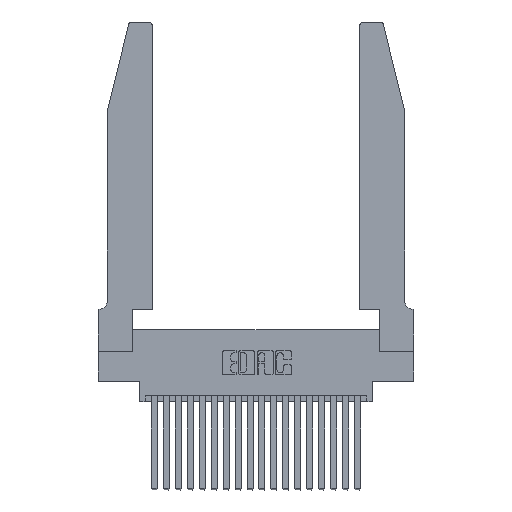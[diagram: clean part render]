
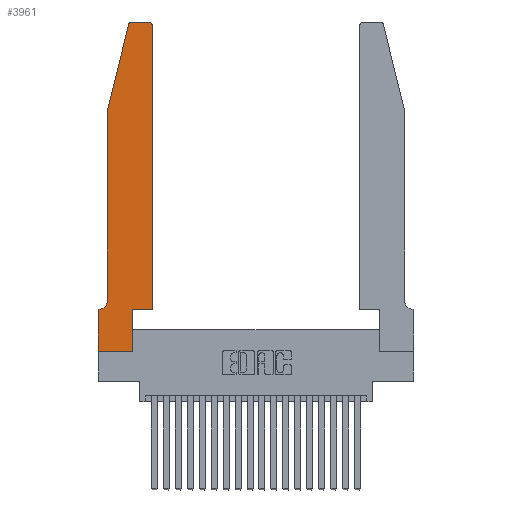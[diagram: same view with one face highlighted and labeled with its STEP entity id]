
A CAD part, top view. The second image highlights one B-rep face of the part: STEP entity #3961.
In plain terms, the highlighted planar face has unit normal (0, 0, 1).
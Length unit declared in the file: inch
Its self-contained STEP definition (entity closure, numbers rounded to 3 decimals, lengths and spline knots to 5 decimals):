
#35 = EDGE_CURVE ( 'NONE', #13079, #6529, #223, .T. ) ;
#199 = DIRECTION ( 'NONE',  ( -0.239, -0.971, 0. ) ) ;
#223 = LINE ( 'NONE', #14886, #17971 ) ;
#735 = CIRCLE ( 'NONE', #3611, 0.07 ) ;
#894 = ORIENTED_EDGE ( 'NONE', *, *, #7632, .T. ) ;
#1057 = VERTEX_POINT ( 'NONE', #8430 ) ;
#1922 = DIRECTION ( 'NONE',  ( -1., 0., 0. ) ) ;
#2214 = LINE ( 'NONE', #8737, #18804 ) ;
#2831 = CARTESIAN_POINT ( 'NONE',  ( 0.2865, 0.35, 0.37 ) ) ;
#2945 = CARTESIAN_POINT ( 'NONE',  ( 0.0755, 2., 0.37 ) ) ;
#3165 = DIRECTION ( 'NONE',  ( 0., 0., 1. ) ) ;
#3611 = AXIS2_PLACEMENT_3D ( 'NONE', #7350, #19250, #9054 ) ;
#3693 = CIRCLE ( 'NONE', #13546, 0.03 ) ;
#3961 = ADVANCED_FACE ( 'NONE', ( #19133 ), #3988, .T. ) ;
#3988 = PLANE ( 'NONE',  #6162 ) ;
#4061 = LINE ( 'NONE', #18383, #12732 ) ;
#4162 = CARTESIAN_POINT ( 'NONE',  ( 0.0055, 0.35, 0.37 ) ) ;
#4624 = CARTESIAN_POINT ( 'NONE',  ( 0., 0., 0.37 ) ) ;
#5386 = CARTESIAN_POINT ( 'NONE',  ( 0.4205, 2.72, 0.37 ) ) ;
#5396 = ORIENTED_EDGE ( 'NONE', *, *, #18853, .T. ) ;
#5871 = CARTESIAN_POINT ( 'NONE',  ( 0.0755, 0.42, 0.37 ) ) ;
#5880 = LINE ( 'NONE', #20763, #18961 ) ;
#6095 = ORIENTED_EDGE ( 'NONE', *, *, #13916, .T. ) ;
#6162 = AXIS2_PLACEMENT_3D ( 'NONE', #16023, #17713, #7493 ) ;
#6344 = EDGE_CURVE ( 'NONE', #21919, #13079, #7239, .T. ) ;
#6529 = VERTEX_POINT ( 'NONE', #12059 ) ;
#6833 = ORIENTED_EDGE ( 'NONE', *, *, #9763, .T. ) ;
#7139 = DIRECTION ( 'NONE',  ( 1., 0., 0. ) ) ;
#7226 = VERTEX_POINT ( 'NONE', #10569 ) ;
#7239 = LINE ( 'NONE', #4624, #15816 ) ;
#7350 = CARTESIAN_POINT ( 'NONE',  ( 0.0055, 0.42, 0.37 ) ) ;
#7493 = DIRECTION ( 'NONE',  ( 1., 0., 0. ) ) ;
#7632 = EDGE_CURVE ( 'NONE', #1057, #8262, #18911, .T. ) ;
#7889 = VERTEX_POINT ( 'NONE', #17749 ) ;
#8262 = VERTEX_POINT ( 'NONE', #20699 ) ;
#8427 = VECTOR ( 'NONE', #17951, 39.37008 ) ;
#8430 = CARTESIAN_POINT ( 'NONE',  ( 0.284, 2.75, 0.37 ) ) ;
#8674 = ORIENTED_EDGE ( 'NONE', *, *, #17031, .T. ) ;
#8737 = CARTESIAN_POINT ( 'NONE',  ( 0.0755, 2., 0.37 ) ) ;
#8948 = CARTESIAN_POINT ( 'NONE',  ( 0.4205, 2.75, 0.37 ) ) ;
#8961 = VERTEX_POINT ( 'NONE', #5871 ) ;
#9054 = DIRECTION ( 'NONE',  ( -1., 0., 0. ) ) ;
#9763 = EDGE_CURVE ( 'NONE', #18347, #1057, #19605, .T. ) ;
#10079 = DIRECTION ( 'NONE',  ( -1., 0., 0. ) ) ;
#10315 = VERTEX_POINT ( 'NONE', #4162 ) ;
#10489 = DIRECTION ( 'NONE',  ( 0., -1., 0. ) ) ;
#10569 = CARTESIAN_POINT ( 'NONE',  ( 0.4505, 0.35, 0.37 ) ) ;
#10728 = LINE ( 'NONE', #18016, #19208 ) ;
#10960 = ORIENTED_EDGE ( 'NONE', *, *, #14172, .T. ) ;
#11254 = EDGE_CURVE ( 'NONE', #21635, #8961, #2214, .T. ) ;
#12022 = ORIENTED_EDGE ( 'NONE', *, *, #6344, .T. ) ;
#12059 = CARTESIAN_POINT ( 'NONE',  ( 0.2865, 0., 0.37 ) ) ;
#12732 = VECTOR ( 'NONE', #21693, 39.37008 ) ;
#13079 = VERTEX_POINT ( 'NONE', #15559 ) ;
#13095 = ORIENTED_EDGE ( 'NONE', *, *, #35, .T. ) ;
#13500 = CARTESIAN_POINT ( 'NONE',  ( 0.284, 2.72, 0.37 ) ) ;
#13546 = AXIS2_PLACEMENT_3D ( 'NONE', #5386, #17365, #7139 ) ;
#13916 = EDGE_CURVE ( 'NONE', #20949, #7226, #21890, .T. ) ;
#14172 = EDGE_CURVE ( 'NONE', #6529, #20949, #4061, .T. ) ;
#14866 = DIRECTION ( 'NONE',  ( 1., 0., 0. ) ) ;
#14886 = CARTESIAN_POINT ( 'NONE',  ( 0., 0., 0.37 ) ) ;
#14949 = DIRECTION ( 'NONE',  ( 0., -1., 0. ) ) ;
#15161 = VECTOR ( 'NONE', #10079, 39.37008 ) ;
#15201 = DIRECTION ( 'NONE',  ( 1., 0., 0. ) ) ;
#15425 = VECTOR ( 'NONE', #199, 39.37008 ) ;
#15559 = CARTESIAN_POINT ( 'NONE',  ( 0., 0., 0.37 ) ) ;
#15682 = ORIENTED_EDGE ( 'NONE', *, *, #19096, .T. ) ;
#15687 = AXIS2_PLACEMENT_3D ( 'NONE', #13500, #3165, #15201 ) ;
#15816 = VECTOR ( 'NONE', #14949, 39.37008 ) ;
#16023 = CARTESIAN_POINT ( 'NONE',  ( 0., 0.35, 0.37 ) ) ;
#16260 = CARTESIAN_POINT ( 'NONE',  ( 0.4505, 0.35, 0.37 ) ) ;
#16568 = ORIENTED_EDGE ( 'NONE', *, *, #18883, .T. ) ;
#17031 = EDGE_CURVE ( 'NONE', #7889, #18347, #3693, .T. ) ;
#17097 = EDGE_LOOP ( 'NONE', ( #6833, #894, #19320, #20086, #16568, #5396, #12022, #13095, #10960, #6095, #15682, #8674 ) ) ;
#17266 = CARTESIAN_POINT ( 'NONE',  ( 0.0755, 2., 0.37 ) ) ;
#17365 = DIRECTION ( 'NONE',  ( 0., 0., 1. ) ) ;
#17713 = DIRECTION ( 'NONE',  ( 0., 0., 1. ) ) ;
#17749 = CARTESIAN_POINT ( 'NONE',  ( 0.4505, 2.72, 0.37 ) ) ;
#17951 = DIRECTION ( 'NONE',  ( 1., 0., 0. ) ) ;
#17971 = VECTOR ( 'NONE', #14866, 39.37008 ) ;
#18016 = CARTESIAN_POINT ( 'NONE',  ( 0.4505, 0.35, 0.37 ) ) ;
#18347 = VERTEX_POINT ( 'NONE', #8948 ) ;
#18383 = CARTESIAN_POINT ( 'NONE',  ( 0.2865, 0.35, 0.37 ) ) ;
#18551 = CARTESIAN_POINT ( 'NONE',  ( 0.2605, 2.75, 0.37 ) ) ;
#18804 = VECTOR ( 'NONE', #10489, 39.37008 ) ;
#18853 = EDGE_CURVE ( 'NONE', #10315, #21919, #5880, .T. ) ;
#18883 = EDGE_CURVE ( 'NONE', #8961, #10315, #735, .T. ) ;
#18911 = CIRCLE ( 'NONE', #15687, 0.03 ) ;
#18961 = VECTOR ( 'NONE', #1922, 39.37008 ) ;
#19096 = EDGE_CURVE ( 'NONE', #7226, #7889, #10728, .T. ) ;
#19133 = FACE_OUTER_BOUND ( 'NONE', #17097, .T. ) ;
#19208 = VECTOR ( 'NONE', #19763, 39.37008 ) ;
#19250 = DIRECTION ( 'NONE',  ( 0., 0., -1. ) ) ;
#19320 = ORIENTED_EDGE ( 'NONE', *, *, #21929, .T. ) ;
#19605 = LINE ( 'NONE', #18551, #15161 ) ;
#19763 = DIRECTION ( 'NONE',  ( 0., 1., 0. ) ) ;
#19873 = LINE ( 'NONE', #17266, #15425 ) ;
#20086 = ORIENTED_EDGE ( 'NONE', *, *, #11254, .T. ) ;
#20680 = CARTESIAN_POINT ( 'NONE',  ( 0., 0.35, 0.37 ) ) ;
#20699 = CARTESIAN_POINT ( 'NONE',  ( 0.25487, 2.72718, 0.37 ) ) ;
#20763 = CARTESIAN_POINT ( 'NONE',  ( 0.0755, 0.35, 0.37 ) ) ;
#20949 = VERTEX_POINT ( 'NONE', #2831 ) ;
#21635 = VERTEX_POINT ( 'NONE', #2945 ) ;
#21693 = DIRECTION ( 'NONE',  ( 0., 1., 0. ) ) ;
#21890 = LINE ( 'NONE', #16260, #8427 ) ;
#21919 = VERTEX_POINT ( 'NONE', #20680 ) ;
#21929 = EDGE_CURVE ( 'NONE', #8262, #21635, #19873, .T. ) ;
